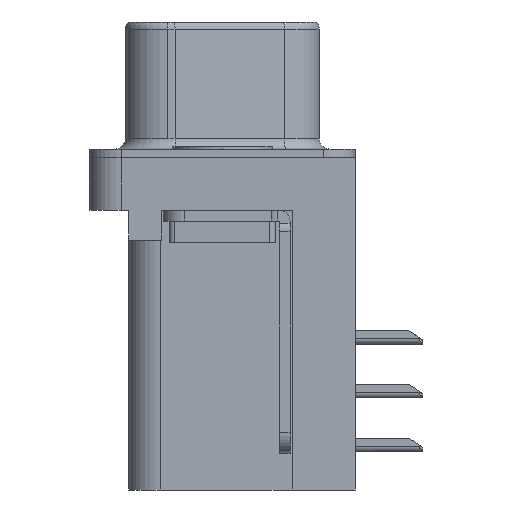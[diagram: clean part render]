
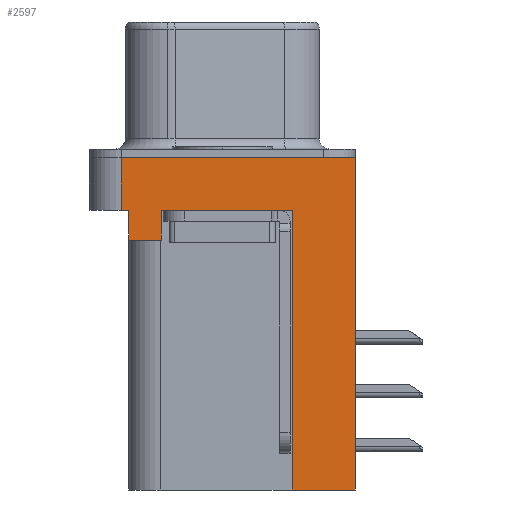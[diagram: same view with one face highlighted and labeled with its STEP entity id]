
A CAD part, left-side view. The second image highlights one B-rep face of the part: STEP entity #2597.
In plain terms, the highlighted planar face has unit normal (-1, 0, 0).
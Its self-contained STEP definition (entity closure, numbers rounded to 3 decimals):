
#12 = DIRECTION ( 'NONE',  ( 0., -1., 0. ) ) ;
#425 = EDGE_CURVE ( 'NONE', #2956, #9389, #570, .T. ) ;
#570 = LINE ( 'NONE', #9384, #8843 ) ;
#1041 = CARTESIAN_POINT ( 'NONE',  ( -2.935, 2.895, -3.9 ) ) ;
#1357 = DIRECTION ( 'NONE',  ( 0., 1., 0. ) ) ;
#1452 = CARTESIAN_POINT ( 'NONE',  ( -2.935, -6.275, -2.5 ) ) ;
#1831 = EDGE_CURVE ( 'NONE', #2956, #3875, #11348, .T. ) ;
#1958 = CARTESIAN_POINT ( 'NONE',  ( -2.935, -6.275, -2.5 ) ) ;
#2269 = ORIENTED_EDGE ( 'NONE', *, *, #12912, .T. ) ;
#2597 = ADVANCED_FACE ( 'NONE', ( #10254 ), #5413, .T. ) ;
#2716 = DIRECTION ( 'NONE',  ( 0., 0., 1. ) ) ;
#2956 = VERTEX_POINT ( 'NONE', #13360 ) ;
#3227 = CARTESIAN_POINT ( 'NONE',  ( -2.935, 4.775, 0. ) ) ;
#3875 = VERTEX_POINT ( 'NONE', #12805 ) ;
#4950 = ORIENTED_EDGE ( 'NONE', *, *, #19315, .F. ) ;
#5413 = PLANE ( 'NONE',  #13161 ) ;
#5514 = ORIENTED_EDGE ( 'NONE', *, *, #19761, .F. ) ;
#5567 = VERTEX_POINT ( 'NONE', #9266 ) ;
#6055 = VECTOR ( 'NONE', #2716, 1000. ) ;
#6358 = EDGE_LOOP ( 'NONE', ( #6434, #19940, #2269, #4950, #15262, #16035, #9598, #5514, #21386, #14589 ) ) ;
#6434 = ORIENTED_EDGE ( 'NONE', *, *, #18187, .F. ) ;
#6684 = DIRECTION ( 'NONE',  ( 0., -1., 0. ) ) ;
#7059 = DIRECTION ( 'NONE',  ( 0., 0., 1. ) ) ;
#7485 = VECTOR ( 'NONE', #7853, 1000. ) ;
#7740 = CARTESIAN_POINT ( 'NONE',  ( -2.935, 4.425, -3.9 ) ) ;
#7853 = DIRECTION ( 'NONE',  ( 0., -1., 0. ) ) ;
#8425 = VERTEX_POINT ( 'NONE', #10750 ) ;
#8575 = VERTEX_POINT ( 'NONE', #19442 ) ;
#8794 = DIRECTION ( 'NONE',  ( 0., 0., 1. ) ) ;
#8843 = VECTOR ( 'NONE', #1357, 1000. ) ;
#9169 = CARTESIAN_POINT ( 'NONE',  ( -2.935, 4.425, -3.9 ) ) ;
#9266 = CARTESIAN_POINT ( 'NONE',  ( -2.935, 4.775, -2.5 ) ) ;
#9381 = DIRECTION ( 'NONE',  ( 0., 1., 0. ) ) ;
#9384 = CARTESIAN_POINT ( 'NONE',  ( -2.935, -3.295, -15.7 ) ) ;
#9389 = VERTEX_POINT ( 'NONE', #14528 ) ;
#9598 = ORIENTED_EDGE ( 'NONE', *, *, #12576, .T. ) ;
#9928 = CARTESIAN_POINT ( 'NONE',  ( -2.935, -6.275, 0. ) ) ;
#9948 = CARTESIAN_POINT ( 'NONE',  ( -2.935, -6.275, -2.5 ) ) ;
#10003 = VECTOR ( 'NONE', #8794, 1000. ) ;
#10254 = FACE_OUTER_BOUND ( 'NONE', #6358, .T. ) ;
#10684 = CARTESIAN_POINT ( 'NONE',  ( -2.935, 4.775, -2.5 ) ) ;
#10750 = CARTESIAN_POINT ( 'NONE',  ( -2.935, -3.295, -2.5 ) ) ;
#11063 = LINE ( 'NONE', #18326, #14944 ) ;
#11348 = LINE ( 'NONE', #1452, #15209 ) ;
#12312 = DIRECTION ( 'NONE',  ( 0., 0., 1. ) ) ;
#12534 = VERTEX_POINT ( 'NONE', #3227 ) ;
#12576 = EDGE_CURVE ( 'NONE', #8575, #8425, #18617, .T. ) ;
#12730 = CARTESIAN_POINT ( 'NONE',  ( -2.935, -6.275, -2.5 ) ) ;
#12782 = LINE ( 'NONE', #7740, #21135 ) ;
#12805 = CARTESIAN_POINT ( 'NONE',  ( -2.935, -6.275, 0. ) ) ;
#12895 = LINE ( 'NONE', #12730, #7485 ) ;
#12912 = EDGE_CURVE ( 'NONE', #5567, #13081, #12895, .T. ) ;
#13081 = VERTEX_POINT ( 'NONE', #19815 ) ;
#13161 = AXIS2_PLACEMENT_3D ( 'NONE', #1958, #16892, #7059 ) ;
#13273 = DIRECTION ( 'NONE',  ( 0., 0., 1. ) ) ;
#13360 = CARTESIAN_POINT ( 'NONE',  ( -2.935, -6.275, -15.7 ) ) ;
#14528 = CARTESIAN_POINT ( 'NONE',  ( -2.935, -3.295, -15.7 ) ) ;
#14589 = ORIENTED_EDGE ( 'NONE', *, *, #1831, .T. ) ;
#14617 = LINE ( 'NONE', #10684, #15146 ) ;
#14944 = VECTOR ( 'NONE', #20041, 1000. ) ;
#15146 = VECTOR ( 'NONE', #12312, 1000. ) ;
#15209 = VECTOR ( 'NONE', #13273, 1000. ) ;
#15248 = VECTOR ( 'NONE', #6684, 1000. ) ;
#15255 = VECTOR ( 'NONE', #12, 1000. ) ;
#15262 = ORIENTED_EDGE ( 'NONE', *, *, #20870, .F. ) ;
#15747 = LINE ( 'NONE', #9928, #15248 ) ;
#15753 = EDGE_CURVE ( 'NONE', #19444, #8575, #20310, .T. ) ;
#16035 = ORIENTED_EDGE ( 'NONE', *, *, #15753, .T. ) ;
#16892 = DIRECTION ( 'NONE',  ( -1., 0., 0. ) ) ;
#17446 = VERTEX_POINT ( 'NONE', #9169 ) ;
#18187 = EDGE_CURVE ( 'NONE', #12534, #3875, #15747, .T. ) ;
#18326 = CARTESIAN_POINT ( 'NONE',  ( -2.935, 4.425, -3.9 ) ) ;
#18617 = LINE ( 'NONE', #9948, #15255 ) ;
#18801 = LINE ( 'NONE', #20428, #10003 ) ;
#19315 = EDGE_CURVE ( 'NONE', #17446, #13081, #11063, .T. ) ;
#19442 = CARTESIAN_POINT ( 'NONE',  ( -2.935, 2.895, -2.5 ) ) ;
#19444 = VERTEX_POINT ( 'NONE', #20954 ) ;
#19761 = EDGE_CURVE ( 'NONE', #9389, #8425, #18801, .T. ) ;
#19815 = CARTESIAN_POINT ( 'NONE',  ( -2.935, 4.425, -2.5 ) ) ;
#19940 = ORIENTED_EDGE ( 'NONE', *, *, #20445, .F. ) ;
#20041 = DIRECTION ( 'NONE',  ( 0., 0., 1. ) ) ;
#20310 = LINE ( 'NONE', #1041, #6055 ) ;
#20428 = CARTESIAN_POINT ( 'NONE',  ( -2.935, -3.295, -15.7 ) ) ;
#20445 = EDGE_CURVE ( 'NONE', #5567, #12534, #14617, .T. ) ;
#20870 = EDGE_CURVE ( 'NONE', #19444, #17446, #12782, .T. ) ;
#20954 = CARTESIAN_POINT ( 'NONE',  ( -2.935, 2.895, -3.9 ) ) ;
#21135 = VECTOR ( 'NONE', #9381, 1000. ) ;
#21386 = ORIENTED_EDGE ( 'NONE', *, *, #425, .F. ) ;
